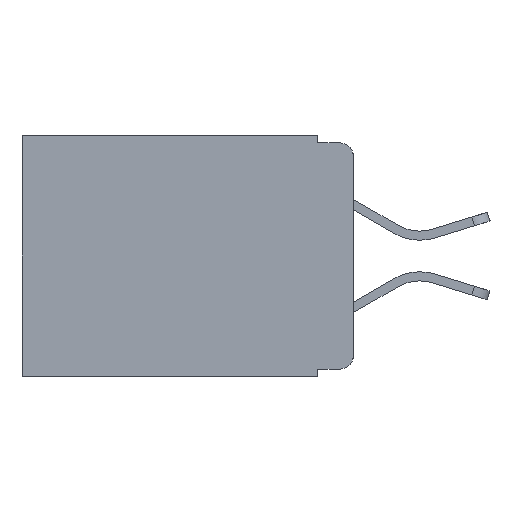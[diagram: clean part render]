
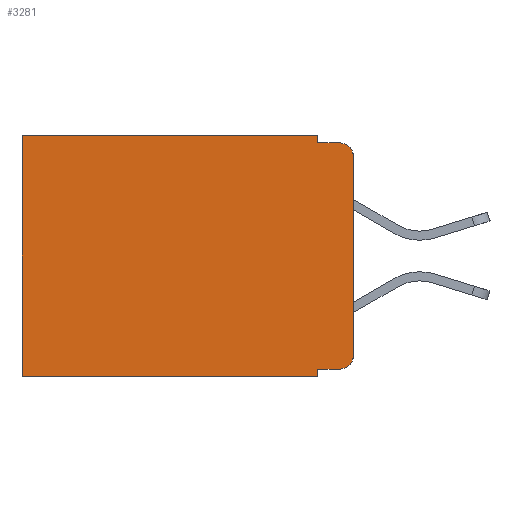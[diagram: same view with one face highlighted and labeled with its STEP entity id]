
A CAD part, left-side view. The second image highlights one B-rep face of the part: STEP entity #3281.
In plain terms, the highlighted planar face has unit normal (-1, 0, 0).
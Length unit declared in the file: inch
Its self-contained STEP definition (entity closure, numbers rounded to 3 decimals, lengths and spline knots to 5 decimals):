
#42 = VECTOR ( 'NONE', #12718, 39.37008 ) ;
#445 = VERTEX_POINT ( 'NONE', #16311 ) ;
#1424 = DIRECTION ( 'NONE',  ( 0., -1., 0. ) ) ;
#1622 = VERTEX_POINT ( 'NONE', #13335 ) ;
#1953 = CARTESIAN_POINT ( 'NONE',  ( 0.298, 0.473, 0. ) ) ;
#2073 = DIRECTION ( 'NONE',  ( -1., 0., 0. ) ) ;
#2475 = VECTOR ( 'NONE', #16108, 39.37008 ) ;
#2676 = ORIENTED_EDGE ( 'NONE', *, *, #18112, .F. ) ;
#3096 = ORIENTED_EDGE ( 'NONE', *, *, #9957, .F. ) ;
#3281 = ADVANCED_FACE ( 'NONE', ( #23037 ), #3393, .F. ) ;
#3393 = PLANE ( 'NONE',  #4844 ) ;
#3531 = DIRECTION ( 'NONE',  ( 0., -1., 0. ) ) ;
#3986 = ORIENTED_EDGE ( 'NONE', *, *, #21127, .F. ) ;
#4302 = AXIS2_PLACEMENT_3D ( 'NONE', #18296, #2073, #18171 ) ;
#4844 = AXIS2_PLACEMENT_3D ( 'NONE', #19836, #6839, #15834 ) ;
#4978 = CARTESIAN_POINT ( 'NONE',  ( 0.298, 0.051, -0.01 ) ) ;
#5098 = LINE ( 'NONE', #4978, #21986 ) ;
#5229 = EDGE_CURVE ( 'NONE', #13934, #12913, #5098, .T. ) ;
#5234 = VECTOR ( 'NONE', #3531, 39.37008 ) ;
#6046 = VERTEX_POINT ( 'NONE', #17250 ) ;
#6156 = CARTESIAN_POINT ( 'NONE',  ( 0.298, 0.051, -0.343 ) ) ;
#6515 = LINE ( 'NONE', #13715, #15813 ) ;
#6618 = EDGE_CURVE ( 'NONE', #23252, #15716, #17259, .T. ) ;
#6678 = CARTESIAN_POINT ( 'NONE',  ( 0.298, 0., 0. ) ) ;
#6839 = DIRECTION ( 'NONE',  ( 1., 0., 0. ) ) ;
#7116 = CARTESIAN_POINT ( 'NONE',  ( 0.298, 0.051, 0. ) ) ;
#7207 = CARTESIAN_POINT ( 'NONE',  ( 0.298, 0.051, -0.333 ) ) ;
#7454 = EDGE_CURVE ( 'NONE', #19623, #20591, #10137, .T. ) ;
#7708 = CIRCLE ( 'NONE', #4302, 0.02 ) ;
#7716 = EDGE_CURVE ( 'NONE', #11076, #12913, #7708, .T. ) ;
#8107 = LINE ( 'NONE', #6678, #10447 ) ;
#8308 = DIRECTION ( 'NONE',  ( 0., 0., -1. ) ) ;
#8884 = CARTESIAN_POINT ( 'NONE',  ( 0.298, 0.02, -0.313 ) ) ;
#9861 = ORIENTED_EDGE ( 'NONE', *, *, #14275, .T. ) ;
#9957 = EDGE_CURVE ( 'NONE', #11076, #15716, #11187, .T. ) ;
#10137 = LINE ( 'NONE', #17368, #22020 ) ;
#10447 = VECTOR ( 'NONE', #12096, 39.37008 ) ;
#10946 = CARTESIAN_POINT ( 'NONE',  ( 0.298, 0., 0. ) ) ;
#11076 = VERTEX_POINT ( 'NONE', #11726 ) ;
#11187 = LINE ( 'NONE', #10946, #42 ) ;
#11241 = ORIENTED_EDGE ( 'NONE', *, *, #7454, .F. ) ;
#11726 = CARTESIAN_POINT ( 'NONE',  ( 0.298, 0., -0.03 ) ) ;
#12096 = DIRECTION ( 'NONE',  ( 0., 1., 0. ) ) ;
#12417 = DIRECTION ( 'NONE',  ( 0., 0., -1. ) ) ;
#12421 = LINE ( 'NONE', #7116, #2475 ) ;
#12718 = DIRECTION ( 'NONE',  ( 0., 0., -1. ) ) ;
#12889 = DIRECTION ( 'NONE',  ( -1., 0., 0. ) ) ;
#12913 = VERTEX_POINT ( 'NONE', #15099 ) ;
#13335 = CARTESIAN_POINT ( 'NONE',  ( 0.298, 0.473, 0. ) ) ;
#13715 = CARTESIAN_POINT ( 'NONE',  ( 0.298, 0.051, 0. ) ) ;
#13934 = VERTEX_POINT ( 'NONE', #22781 ) ;
#14275 = EDGE_CURVE ( 'NONE', #6046, #1622, #8107, .T. ) ;
#14603 = LINE ( 'NONE', #1953, #16415 ) ;
#15099 = CARTESIAN_POINT ( 'NONE',  ( 0.298, 0.02, -0.01 ) ) ;
#15211 = ORIENTED_EDGE ( 'NONE', *, *, #21274, .T. ) ;
#15224 = EDGE_CURVE ( 'NONE', #1622, #20591, #14603, .T. ) ;
#15588 = DIRECTION ( 'NONE',  ( 0., 1., 0. ) ) ;
#15624 = ORIENTED_EDGE ( 'NONE', *, *, #5229, .F. ) ;
#15646 = ORIENTED_EDGE ( 'NONE', *, *, #6618, .T. ) ;
#15716 = VERTEX_POINT ( 'NONE', #22526 ) ;
#15813 = VECTOR ( 'NONE', #8308, 39.37008 ) ;
#15834 = DIRECTION ( 'NONE',  ( 0., 0., -1. ) ) ;
#15970 = LINE ( 'NONE', #7207, #5234 ) ;
#16108 = DIRECTION ( 'NONE',  ( 0., 0., -1. ) ) ;
#16311 = CARTESIAN_POINT ( 'NONE',  ( 0.298, 0.051, -0.333 ) ) ;
#16415 = VECTOR ( 'NONE', #19932, 39.37008 ) ;
#17249 = ORIENTED_EDGE ( 'NONE', *, *, #15224, .T. ) ;
#17250 = CARTESIAN_POINT ( 'NONE',  ( 0.298, 0.051, 0. ) ) ;
#17259 = CIRCLE ( 'NONE', #19139, 0.02 ) ;
#17368 = CARTESIAN_POINT ( 'NONE',  ( 0.298, 0., -0.343 ) ) ;
#18112 = EDGE_CURVE ( 'NONE', #6046, #13934, #12421, .T. ) ;
#18171 = DIRECTION ( 'NONE',  ( 0., 0., -1. ) ) ;
#18296 = CARTESIAN_POINT ( 'NONE',  ( 0.298, 0.02, -0.03 ) ) ;
#18860 = CARTESIAN_POINT ( 'NONE',  ( 0.298, 0.02, -0.333 ) ) ;
#18971 = ORIENTED_EDGE ( 'NONE', *, *, #7716, .T. ) ;
#19139 = AXIS2_PLACEMENT_3D ( 'NONE', #8884, #12889, #12417 ) ;
#19623 = VERTEX_POINT ( 'NONE', #6156 ) ;
#19836 = CARTESIAN_POINT ( 'NONE',  ( 0.298, 0., 0. ) ) ;
#19932 = DIRECTION ( 'NONE',  ( 0., 0., -1. ) ) ;
#20520 = CARTESIAN_POINT ( 'NONE',  ( 0.298, 0.473, -0.343 ) ) ;
#20537 = EDGE_LOOP ( 'NONE', ( #3096, #18971, #15624, #2676, #9861, #17249, #11241, #3986, #15211, #15646 ) ) ;
#20591 = VERTEX_POINT ( 'NONE', #20520 ) ;
#21127 = EDGE_CURVE ( 'NONE', #445, #19623, #6515, .T. ) ;
#21274 = EDGE_CURVE ( 'NONE', #445, #23252, #15970, .T. ) ;
#21986 = VECTOR ( 'NONE', #1424, 39.37008 ) ;
#22020 = VECTOR ( 'NONE', #15588, 39.37008 ) ;
#22526 = CARTESIAN_POINT ( 'NONE',  ( 0.298, 0., -0.313 ) ) ;
#22781 = CARTESIAN_POINT ( 'NONE',  ( 0.298, 0.051, -0.01 ) ) ;
#23037 = FACE_OUTER_BOUND ( 'NONE', #20537, .T. ) ;
#23252 = VERTEX_POINT ( 'NONE', #18860 ) ;
